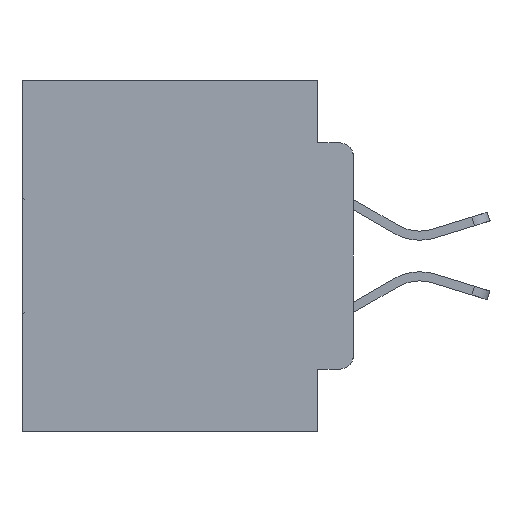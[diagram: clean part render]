
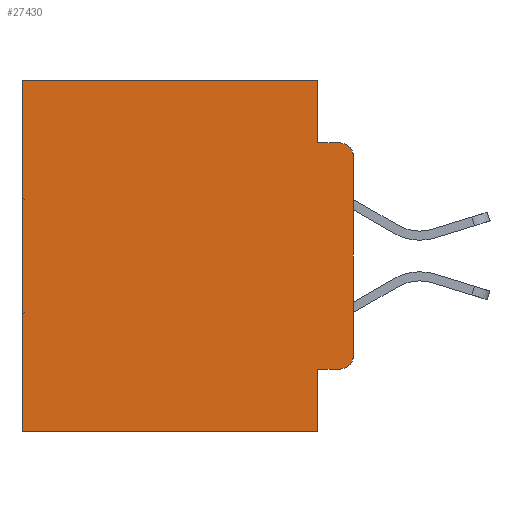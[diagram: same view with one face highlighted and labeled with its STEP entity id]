
A CAD part, left-side view. The second image highlights one B-rep face of the part: STEP entity #27430.
In plain terms, the highlighted planar face has unit normal (-1, 0, 0).
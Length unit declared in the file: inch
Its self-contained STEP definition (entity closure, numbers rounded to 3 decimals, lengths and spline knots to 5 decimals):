
#89 = ORIENTED_EDGE ( 'NONE', *, *, #17477, .F. ) ;
#855 = CARTESIAN_POINT ( 'NONE',  ( 0.298, 0.051, -0.0885 ) ) ;
#1166 = EDGE_CURVE ( 'NONE', #6518, #21458, #1993, .T. ) ;
#1315 = DIRECTION ( 'NONE',  ( -1., 0., 0. ) ) ;
#1609 = AXIS2_PLACEMENT_3D ( 'NONE', #25773, #1315, #28328 ) ;
#1831 = CARTESIAN_POINT ( 'NONE',  ( 0.298, 0., -0.3915 ) ) ;
#1993 = CIRCLE ( 'NONE', #9817, 0.02 ) ;
#2134 = CARTESIAN_POINT ( 'NONE',  ( 0.298, 0.051, -0.4115 ) ) ;
#2578 = EDGE_LOOP ( 'NONE', ( #30427, #5587, #89, #30690, #26958, #11604, #4448, #27987, #9107, #28963 ) ) ;
#3466 = DIRECTION ( 'NONE',  ( 1., 0., 0. ) ) ;
#3852 = VECTOR ( 'NONE', #28422, 39.37008 ) ;
#3860 = VECTOR ( 'NONE', #29640, 39.37008 ) ;
#4184 = EDGE_CURVE ( 'NONE', #13554, #27277, #21638, .T. ) ;
#4448 = ORIENTED_EDGE ( 'NONE', *, *, #7067, .F. ) ;
#4669 = CARTESIAN_POINT ( 'NONE',  ( 0.298, 0., 0. ) ) ;
#5387 = LINE ( 'NONE', #6462, #3852 ) ;
#5587 = ORIENTED_EDGE ( 'NONE', *, *, #4184, .T. ) ;
#6162 = CARTESIAN_POINT ( 'NONE',  ( 0.298, 0., 0. ) ) ;
#6453 = LINE ( 'NONE', #855, #11438 ) ;
#6462 = CARTESIAN_POINT ( 'NONE',  ( 0.298, 0., 0. ) ) ;
#6518 = VERTEX_POINT ( 'NONE', #7813 ) ;
#7067 = EDGE_CURVE ( 'NONE', #22686, #17094, #28731, .T. ) ;
#7813 = CARTESIAN_POINT ( 'NONE',  ( 0.298, 0.02, -0.4115 ) ) ;
#8232 = CARTESIAN_POINT ( 'NONE',  ( 0.298, 0.473, 0. ) ) ;
#8632 = DIRECTION ( 'NONE',  ( 0., 0., -1. ) ) ;
#9008 = VERTEX_POINT ( 'NONE', #8232 ) ;
#9107 = ORIENTED_EDGE ( 'NONE', *, *, #31041, .T. ) ;
#9499 = CARTESIAN_POINT ( 'NONE',  ( 0.298, 0.051, 0. ) ) ;
#9669 = EDGE_CURVE ( 'NONE', #13554, #21458, #5387, .T. ) ;
#9817 = AXIS2_PLACEMENT_3D ( 'NONE', #10321, #12908, #30023 ) ;
#10285 = AXIS2_PLACEMENT_3D ( 'NONE', #6162, #3466, #13266 ) ;
#10321 = CARTESIAN_POINT ( 'NONE',  ( 0.298, 0.02, -0.3915 ) ) ;
#11438 = VECTOR ( 'NONE', #25343, 39.37008 ) ;
#11604 = ORIENTED_EDGE ( 'NONE', *, *, #15937, .T. ) ;
#11755 = DIRECTION ( 'NONE',  ( 0., 0., -1. ) ) ;
#12523 = CARTESIAN_POINT ( 'NONE',  ( 0.298, 0.051, -0.4115 ) ) ;
#12630 = VECTOR ( 'NONE', #19840, 39.37008 ) ;
#12908 = DIRECTION ( 'NONE',  ( -1., 0., 0. ) ) ;
#13266 = DIRECTION ( 'NONE',  ( 0., 0., -1. ) ) ;
#13554 = VERTEX_POINT ( 'NONE', #29283 ) ;
#14166 = LINE ( 'NONE', #4669, #12630 ) ;
#14187 = VECTOR ( 'NONE', #15866, 39.37008 ) ;
#14609 = VECTOR ( 'NONE', #23752, 39.37008 ) ;
#15376 = CARTESIAN_POINT ( 'NONE',  ( 0.298, 0.02, -0.0885 ) ) ;
#15866 = DIRECTION ( 'NONE',  ( 0., 1., 0. ) ) ;
#15902 = PLANE ( 'NONE',  #10285 ) ;
#15937 = EDGE_CURVE ( 'NONE', #9008, #17094, #24615, .T. ) ;
#17058 = CARTESIAN_POINT ( 'NONE',  ( 0.298, 0.051, 0. ) ) ;
#17094 = VERTEX_POINT ( 'NONE', #28226 ) ;
#17477 = EDGE_CURVE ( 'NONE', #19928, #27277, #6453, .T. ) ;
#18062 = CARTESIAN_POINT ( 'NONE',  ( 0.298, 0., -0.5 ) ) ;
#19095 = CARTESIAN_POINT ( 'NONE',  ( 0.298, 0.051, -0.0885 ) ) ;
#19728 = FACE_OUTER_BOUND ( 'NONE', #2578, .T. ) ;
#19840 = DIRECTION ( 'NONE',  ( 0., 1., 0. ) ) ;
#19928 = VERTEX_POINT ( 'NONE', #19095 ) ;
#20654 = VERTEX_POINT ( 'NONE', #2134 ) ;
#21458 = VERTEX_POINT ( 'NONE', #1831 ) ;
#21638 = CIRCLE ( 'NONE', #1609, 0.02 ) ;
#22686 = VERTEX_POINT ( 'NONE', #25783 ) ;
#23752 = DIRECTION ( 'NONE',  ( 0., 0., -1. ) ) ;
#24344 = VECTOR ( 'NONE', #8632, 39.37008 ) ;
#24449 = EDGE_CURVE ( 'NONE', #26786, #9008, #14166, .T. ) ;
#24615 = LINE ( 'NONE', #26059, #14609 ) ;
#24772 = EDGE_CURVE ( 'NONE', #20654, #22686, #26380, .T. ) ;
#25343 = DIRECTION ( 'NONE',  ( 0., -1., 0. ) ) ;
#25463 = CARTESIAN_POINT ( 'NONE',  ( 0.298, 0.051, 0. ) ) ;
#25773 = CARTESIAN_POINT ( 'NONE',  ( 0.298, 0.02, -0.1085 ) ) ;
#25783 = CARTESIAN_POINT ( 'NONE',  ( 0.298, 0.051, -0.5 ) ) ;
#26059 = CARTESIAN_POINT ( 'NONE',  ( 0.298, 0.473, 0. ) ) ;
#26380 = LINE ( 'NONE', #9499, #27143 ) ;
#26786 = VERTEX_POINT ( 'NONE', #17058 ) ;
#26958 = ORIENTED_EDGE ( 'NONE', *, *, #24449, .T. ) ;
#27143 = VECTOR ( 'NONE', #11755, 39.37008 ) ;
#27277 = VERTEX_POINT ( 'NONE', #15376 ) ;
#27385 = EDGE_CURVE ( 'NONE', #26786, #19928, #29274, .T. ) ;
#27430 = ADVANCED_FACE ( 'NONE', ( #19728 ), #15902, .F. ) ;
#27987 = ORIENTED_EDGE ( 'NONE', *, *, #24772, .F. ) ;
#28226 = CARTESIAN_POINT ( 'NONE',  ( 0.298, 0.473, -0.5 ) ) ;
#28328 = DIRECTION ( 'NONE',  ( 0., 0., -1. ) ) ;
#28422 = DIRECTION ( 'NONE',  ( 0., 0., -1. ) ) ;
#28731 = LINE ( 'NONE', #18062, #14187 ) ;
#28963 = ORIENTED_EDGE ( 'NONE', *, *, #1166, .T. ) ;
#29274 = LINE ( 'NONE', #25463, #24344 ) ;
#29283 = CARTESIAN_POINT ( 'NONE',  ( 0.298, 0., -0.1085 ) ) ;
#29553 = LINE ( 'NONE', #12523, #3860 ) ;
#29640 = DIRECTION ( 'NONE',  ( 0., -1., 0. ) ) ;
#30023 = DIRECTION ( 'NONE',  ( 0., 0., -1. ) ) ;
#30427 = ORIENTED_EDGE ( 'NONE', *, *, #9669, .F. ) ;
#30690 = ORIENTED_EDGE ( 'NONE', *, *, #27385, .F. ) ;
#31041 = EDGE_CURVE ( 'NONE', #20654, #6518, #29553, .T. ) ;
